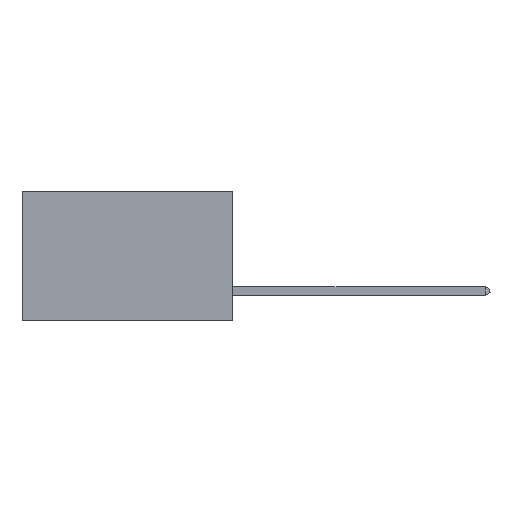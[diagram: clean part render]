
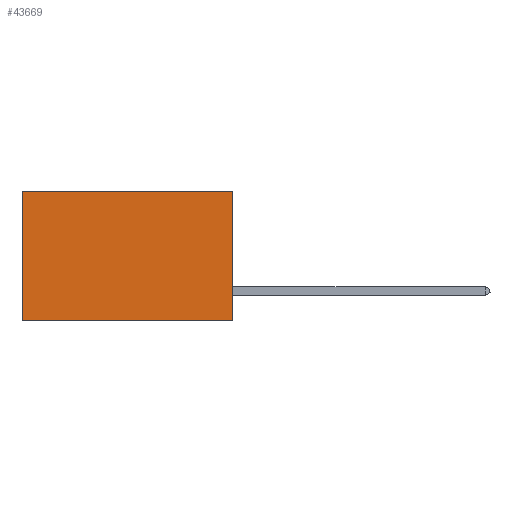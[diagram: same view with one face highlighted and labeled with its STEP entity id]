
A CAD part, left-side view. The second image highlights one B-rep face of the part: STEP entity #43669.
In plain terms, the highlighted planar face has unit normal (-1, 0, 0).
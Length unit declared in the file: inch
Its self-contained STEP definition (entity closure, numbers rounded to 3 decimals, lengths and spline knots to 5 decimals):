
#1073 = LINE ( 'NONE', #47232, #17825 ) ;
#4232 = CARTESIAN_POINT ( 'NONE',  ( 0.2875, 0., 0. ) ) ;
#10645 = EDGE_CURVE ( 'NONE', #21725, #25557, #42839, .T. ) ;
#11163 = ORIENTED_EDGE ( 'NONE', *, *, #34710, .T. ) ;
#12179 = CARTESIAN_POINT ( 'NONE',  ( 0.2875, 0., -0.37 ) ) ;
#12358 = CARTESIAN_POINT ( 'NONE',  ( 0.2875, 0.6, 0. ) ) ;
#14447 = CARTESIAN_POINT ( 'NONE',  ( 0.2875, 0., -0.37 ) ) ;
#14550 = EDGE_CURVE ( 'NONE', #46210, #19582, #1073, .T. ) ;
#14963 = DIRECTION ( 'NONE',  ( 0., 1., 0. ) ) ;
#15534 = LINE ( 'NONE', #14447, #48554 ) ;
#17825 = VECTOR ( 'NONE', #24207, 39.37008 ) ;
#18043 = CARTESIAN_POINT ( 'NONE',  ( 0.2875, 0., 0. ) ) ;
#19098 = CARTESIAN_POINT ( 'NONE',  ( 0.2875, 0.6, 0. ) ) ;
#19302 = ORIENTED_EDGE ( 'NONE', *, *, #33657, .F. ) ;
#19333 = FACE_OUTER_BOUND ( 'NONE', #23129, .T. ) ;
#19582 = VERTEX_POINT ( 'NONE', #12179 ) ;
#21725 = VERTEX_POINT ( 'NONE', #12358 ) ;
#21896 = DIRECTION ( 'NONE',  ( 0., 0., -1. ) ) ;
#23129 = EDGE_LOOP ( 'NONE', ( #31727, #19302, #35277, #11163 ) ) ;
#24207 = DIRECTION ( 'NONE',  ( 0., 0., -1. ) ) ;
#25557 = VERTEX_POINT ( 'NONE', #35120 ) ;
#26520 = AXIS2_PLACEMENT_3D ( 'NONE', #4232, #41019, #21896 ) ;
#31727 = ORIENTED_EDGE ( 'NONE', *, *, #10645, .T. ) ;
#32207 = LINE ( 'NONE', #33408, #35842 ) ;
#33408 = CARTESIAN_POINT ( 'NONE',  ( 0.2875, 0., 0. ) ) ;
#33657 = EDGE_CURVE ( 'NONE', #19582, #25557, #15534, .T. ) ;
#34710 = EDGE_CURVE ( 'NONE', #46210, #21725, #32207, .T. ) ;
#35120 = CARTESIAN_POINT ( 'NONE',  ( 0.2875, 0.6, -0.37 ) ) ;
#35277 = ORIENTED_EDGE ( 'NONE', *, *, #14550, .F. ) ;
#35842 = VECTOR ( 'NONE', #14963, 39.37008 ) ;
#38343 = PLANE ( 'NONE',  #26520 ) ;
#41019 = DIRECTION ( 'NONE',  ( 1., 0., 0. ) ) ;
#42839 = LINE ( 'NONE', #19098, #49495 ) ;
#43669 = ADVANCED_FACE ( 'NONE', ( #19333 ), #38343, .F. ) ;
#45305 = DIRECTION ( 'NONE',  ( 0., 1., 0. ) ) ;
#45452 = DIRECTION ( 'NONE',  ( 0., 0., -1. ) ) ;
#46210 = VERTEX_POINT ( 'NONE', #18043 ) ;
#47232 = CARTESIAN_POINT ( 'NONE',  ( 0.2875, 0., 0. ) ) ;
#48554 = VECTOR ( 'NONE', #45305, 39.37008 ) ;
#49495 = VECTOR ( 'NONE', #45452, 39.37008 ) ;
